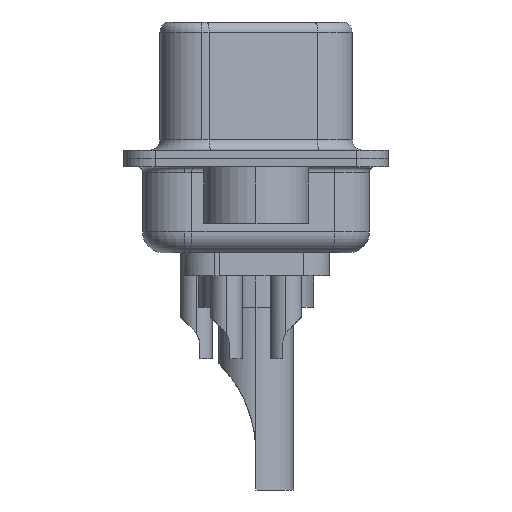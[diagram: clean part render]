
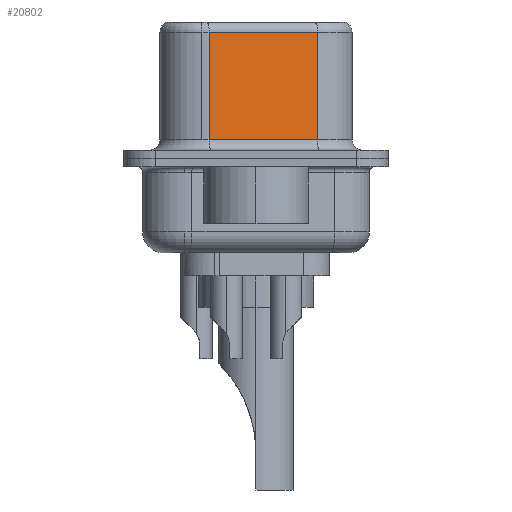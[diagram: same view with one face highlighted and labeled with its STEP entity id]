
A CAD part, left-side view. The second image highlights one B-rep face of the part: STEP entity #20802.
In plain terms, the highlighted planar face has unit normal (-0.985, -0.174, 0).
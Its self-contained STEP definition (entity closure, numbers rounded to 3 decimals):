
#1278 = VERTEX_POINT ( 'NONE', #19052 ) ;
#1350 = DIRECTION ( 'NONE',  ( -0.174, 0.985, 0. ) ) ;
#1841 = DIRECTION ( 'NONE',  ( -0.174, 0.985, 0. ) ) ;
#1857 = CARTESIAN_POINT ( 'NONE',  ( 4.585, -2.927, 6.02 ) ) ;
#1866 = ORIENTED_EDGE ( 'NONE', *, *, #15424, .T. ) ;
#1968 = CARTESIAN_POINT ( 'NONE',  ( 3.675, 2.233, 6.52 ) ) ;
#2065 = EDGE_CURVE ( 'NONE', #4082, #4125, #20878, .T. ) ;
#3164 = VECTOR ( 'NONE', #6636, 1000. ) ;
#3556 = ORIENTED_EDGE ( 'NONE', *, *, #16867, .T. ) ;
#3603 = CARTESIAN_POINT ( 'NONE',  ( 3.675, 2.233, 0.9 ) ) ;
#3699 = LINE ( 'NONE', #20715, #8462 ) ;
#4082 = VERTEX_POINT ( 'NONE', #1857 ) ;
#4125 = VERTEX_POINT ( 'NONE', #17727 ) ;
#6636 = DIRECTION ( 'NONE',  ( 0., 0., -1. ) ) ;
#6880 = DIRECTION ( 'NONE',  ( 0., 0., -1. ) ) ;
#7460 = AXIS2_PLACEMENT_3D ( 'NONE', #17473, #19307, #1350 ) ;
#7979 = PLANE ( 'NONE',  #7460 ) ;
#8351 = ORIENTED_EDGE ( 'NONE', *, *, #2065, .F. ) ;
#8462 = VECTOR ( 'NONE', #18942, 1000. ) ;
#10525 = VERTEX_POINT ( 'NONE', #3603 ) ;
#11633 = CARTESIAN_POINT ( 'NONE',  ( 4.585, -2.927, 6.02 ) ) ;
#13438 = VECTOR ( 'NONE', #1841, 1000. ) ;
#14743 = ORIENTED_EDGE ( 'NONE', *, *, #19832, .T. ) ;
#15416 = CARTESIAN_POINT ( 'NONE',  ( 4.585, -2.927, 6.52 ) ) ;
#15424 = EDGE_CURVE ( 'NONE', #1278, #10525, #19373, .T. ) ;
#16188 = LINE ( 'NONE', #11633, #13438 ) ;
#16867 = EDGE_CURVE ( 'NONE', #10525, #4125, #3699, .T. ) ;
#17085 = VECTOR ( 'NONE', #6880, 1000. ) ;
#17176 = FACE_OUTER_BOUND ( 'NONE', #17267, .T. ) ;
#17267 = EDGE_LOOP ( 'NONE', ( #8351, #14743, #1866, #3556 ) ) ;
#17473 = CARTESIAN_POINT ( 'NONE',  ( 4.585, -2.927, 6.52 ) ) ;
#17727 = CARTESIAN_POINT ( 'NONE',  ( 4.585, -2.927, 0.9 ) ) ;
#18942 = DIRECTION ( 'NONE',  ( 0.174, -0.985, 0. ) ) ;
#19052 = CARTESIAN_POINT ( 'NONE',  ( 3.675, 2.233, 6.02 ) ) ;
#19307 = DIRECTION ( 'NONE',  ( 0.985, 0.174, 0. ) ) ;
#19373 = LINE ( 'NONE', #1968, #3164 ) ;
#19832 = EDGE_CURVE ( 'NONE', #4082, #1278, #16188, .T. ) ;
#20715 = CARTESIAN_POINT ( 'NONE',  ( 4.585, -2.927, 0.9 ) ) ;
#20802 = ADVANCED_FACE ( 'NONE', ( #17176 ), #7979, .F. ) ;
#20878 = LINE ( 'NONE', #15416, #17085 ) ;
